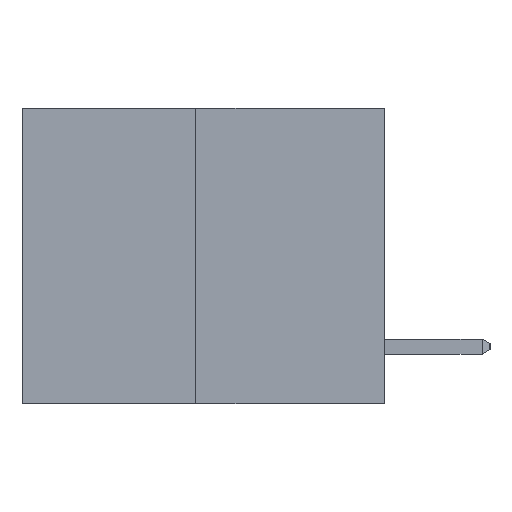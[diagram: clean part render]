
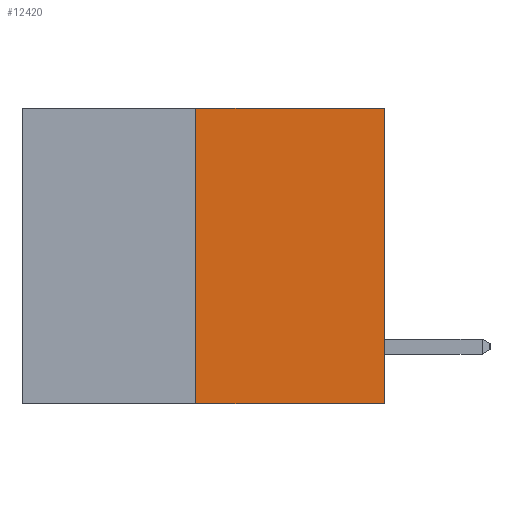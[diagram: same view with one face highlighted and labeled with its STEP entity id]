
A CAD part, left-side view. The second image highlights one B-rep face of the part: STEP entity #12420.
In plain terms, the highlighted planar face has unit normal (-1, 0, 0).
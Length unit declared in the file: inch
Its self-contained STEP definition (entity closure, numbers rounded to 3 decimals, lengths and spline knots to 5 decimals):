
#99 = PLANE ( 'NONE',  #10236 ) ;
#155 = LINE ( 'NONE', #1536, #3147 ) ;
#588 = LINE ( 'NONE', #7963, #10494 ) ;
#1099 = DIRECTION ( 'NONE',  ( 1., 0., 0. ) ) ;
#1458 = DIRECTION ( 'NONE',  ( 0., -1., 0. ) ) ;
#1536 = CARTESIAN_POINT ( 'NONE',  ( 0., 0., 0. ) ) ;
#1869 = ORIENTED_EDGE ( 'NONE', *, *, #10097, .T. ) ;
#2638 = EDGE_LOOP ( 'NONE', ( #7804, #12291, #1869, #12430 ) ) ;
#3090 = DIRECTION ( 'NONE',  ( 0., -1., 0. ) ) ;
#3147 = VECTOR ( 'NONE', #8238, 39.37008 ) ;
#3452 = VECTOR ( 'NONE', #1458, 39.37008 ) ;
#3878 = VECTOR ( 'NONE', #9472, 39.37008 ) ;
#4360 = LINE ( 'NONE', #10212, #3452 ) ;
#4875 = CARTESIAN_POINT ( 'NONE',  ( 0., 0.312, 0. ) ) ;
#5242 = LINE ( 'NONE', #11300, #3878 ) ;
#6293 = FACE_OUTER_BOUND ( 'NONE', #2638, .T. ) ;
#6487 = VERTEX_POINT ( 'NONE', #6737 ) ;
#6737 = CARTESIAN_POINT ( 'NONE',  ( 0., 0., -0.49 ) ) ;
#6828 = CARTESIAN_POINT ( 'NONE',  ( 0., 0.6, 0. ) ) ;
#7037 = CARTESIAN_POINT ( 'NONE',  ( 0., 0.312, -0.49 ) ) ;
#7205 = VERTEX_POINT ( 'NONE', #7037 ) ;
#7537 = VERTEX_POINT ( 'NONE', #4875 ) ;
#7636 = EDGE_CURVE ( 'NONE', #7205, #6487, #588, .T. ) ;
#7804 = ORIENTED_EDGE ( 'NONE', *, *, #12277, .F. ) ;
#7963 = CARTESIAN_POINT ( 'NONE',  ( 0., 0.6, -0.49 ) ) ;
#8238 = DIRECTION ( 'NONE',  ( 0., 0., 1. ) ) ;
#8754 = DIRECTION ( 'NONE',  ( 0., 0., -1. ) ) ;
#9472 = DIRECTION ( 'NONE',  ( 0., 0., 1. ) ) ;
#10079 = EDGE_CURVE ( 'NONE', #7537, #12172, #4360, .T. ) ;
#10097 = EDGE_CURVE ( 'NONE', #6487, #12172, #155, .T. ) ;
#10212 = CARTESIAN_POINT ( 'NONE',  ( 0., 0.6, 0. ) ) ;
#10236 = AXIS2_PLACEMENT_3D ( 'NONE', #6828, #1099, #8754 ) ;
#10494 = VECTOR ( 'NONE', #3090, 39.37008 ) ;
#10516 = CARTESIAN_POINT ( 'NONE',  ( 0., 0., 0. ) ) ;
#11300 = CARTESIAN_POINT ( 'NONE',  ( 0., 0.312, -0.49 ) ) ;
#12172 = VERTEX_POINT ( 'NONE', #10516 ) ;
#12277 = EDGE_CURVE ( 'NONE', #7205, #7537, #5242, .T. ) ;
#12291 = ORIENTED_EDGE ( 'NONE', *, *, #7636, .T. ) ;
#12420 = ADVANCED_FACE ( 'NONE', ( #6293 ), #99, .F. ) ;
#12430 = ORIENTED_EDGE ( 'NONE', *, *, #10079, .F. ) ;
